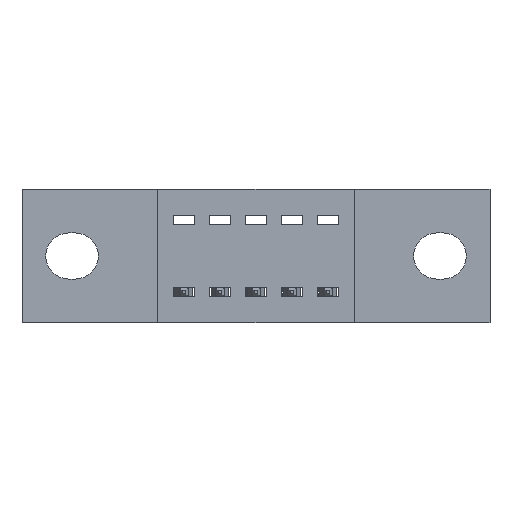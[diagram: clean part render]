
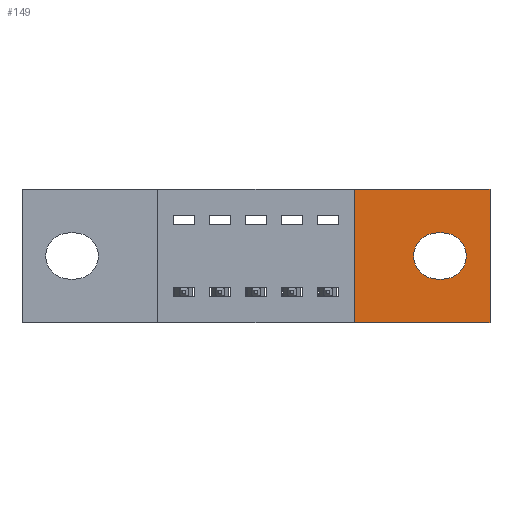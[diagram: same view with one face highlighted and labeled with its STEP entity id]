
A CAD part, front view. The second image highlights one B-rep face of the part: STEP entity #149.
In plain terms, the highlighted planar face has unit normal (0, -1, 0).
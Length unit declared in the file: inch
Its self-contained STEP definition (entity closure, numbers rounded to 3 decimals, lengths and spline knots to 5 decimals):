
#11 = DIRECTION ( 'NONE',  ( -1., 0., 0. ) ) ;
#149 = ADVANCED_FACE ( 'NONE', ( #6236, #7742 ), #6821, .T. ) ;
#252 = LINE ( 'NONE', #1247, #6644 ) ;
#316 = ORIENTED_EDGE ( 'NONE', *, *, #7622, .F. ) ;
#516 = CARTESIAN_POINT ( 'NONE',  ( 1.152, 0., -0.121 ) ) ;
#649 = AXIS2_PLACEMENT_3D ( 'NONE', #7775, #7868, #7463 ) ;
#774 = EDGE_CURVE ( 'NONE', #3691, #2990, #3386, .T. ) ;
#1015 = DIRECTION ( 'NONE',  ( 1., 0., 0. ) ) ;
#1027 = ORIENTED_EDGE ( 'NONE', *, *, #774, .T. ) ;
#1077 = EDGE_CURVE ( 'NONE', #6500, #5155, #3284, .T. ) ;
#1083 = VECTOR ( 'NONE', #11, 39.37008 ) ;
#1247 = CARTESIAN_POINT ( 'NONE',  ( 1.17, 0., -0.249 ) ) ;
#1268 = DIRECTION ( 'NONE',  ( -1., 0., 0. ) ) ;
#1325 = VECTOR ( 'NONE', #3061, 39.37008 ) ;
#1450 = CARTESIAN_POINT ( 'NONE',  ( 1.17, 0., -0.121 ) ) ;
#1493 = VECTOR ( 'NONE', #1015, 39.37008 ) ;
#1642 = CIRCLE ( 'NONE', #7330, 0.064 ) ;
#1705 = DIRECTION ( 'NONE',  ( 0., 0., 1. ) ) ;
#1780 = ORIENTED_EDGE ( 'NONE', *, *, #4935, .F. ) ;
#2041 = CARTESIAN_POINT ( 'NONE',  ( 0.923, 0., 0. ) ) ;
#2083 = VERTEX_POINT ( 'NONE', #2868 ) ;
#2131 = EDGE_CURVE ( 'NONE', #5155, #2083, #2318, .T. ) ;
#2318 = LINE ( 'NONE', #4399, #3565 ) ;
#2379 = CARTESIAN_POINT ( 'NONE',  ( 1.17, 0., -0.185 ) ) ;
#2868 = CARTESIAN_POINT ( 'NONE',  ( 1.3, 0., 0. ) ) ;
#2923 = EDGE_LOOP ( 'NONE', ( #1027, #7491, #4480, #3009 ) ) ;
#2990 = VERTEX_POINT ( 'NONE', #3347 ) ;
#3009 = ORIENTED_EDGE ( 'NONE', *, *, #3537, .T. ) ;
#3061 = DIRECTION ( 'NONE',  ( 0., 0., -1. ) ) ;
#3091 = CARTESIAN_POINT ( 'NONE',  ( 1.3, 0., 0. ) ) ;
#3123 = LINE ( 'NONE', #3091, #1325 ) ;
#3284 = LINE ( 'NONE', #5162, #6405 ) ;
#3317 = EDGE_LOOP ( 'NONE', ( #7819, #1780, #316, #3596 ) ) ;
#3347 = CARTESIAN_POINT ( 'NONE',  ( 1.17, 0., -0.249 ) ) ;
#3386 = CIRCLE ( 'NONE', #7445, 0.064 ) ;
#3406 = VERTEX_POINT ( 'NONE', #7368 ) ;
#3473 = VERTEX_POINT ( 'NONE', #516 ) ;
#3537 = EDGE_CURVE ( 'NONE', #3473, #3691, #7882, .T. ) ;
#3565 = VECTOR ( 'NONE', #6577, 39.37008 ) ;
#3577 = CARTESIAN_POINT ( 'NONE',  ( 0., 0., -0.37 ) ) ;
#3596 = ORIENTED_EDGE ( 'NONE', *, *, #2131, .F. ) ;
#3691 = VERTEX_POINT ( 'NONE', #6468 ) ;
#4213 = DIRECTION ( 'NONE',  ( 0., 1., 0. ) ) ;
#4399 = CARTESIAN_POINT ( 'NONE',  ( 0., 0., 0. ) ) ;
#4420 = CARTESIAN_POINT ( 'NONE',  ( 1.3, 0., -0.37 ) ) ;
#4480 = ORIENTED_EDGE ( 'NONE', *, *, #5614, .T. ) ;
#4597 = DIRECTION ( 'NONE',  ( 0., 0., -1. ) ) ;
#4606 = DIRECTION ( 'NONE',  ( 0., 1., 0. ) ) ;
#4608 = CARTESIAN_POINT ( 'NONE',  ( 1.152, 0., -0.185 ) ) ;
#4642 = CARTESIAN_POINT ( 'NONE',  ( 0.923, 0., -0.37 ) ) ;
#4935 = EDGE_CURVE ( 'NONE', #7365, #6500, #7540, .T. ) ;
#5155 = VERTEX_POINT ( 'NONE', #2041 ) ;
#5162 = CARTESIAN_POINT ( 'NONE',  ( 0.923, 0., -0.37 ) ) ;
#5573 = DIRECTION ( 'NONE',  ( 0., 0., -1. ) ) ;
#5614 = EDGE_CURVE ( 'NONE', #3406, #3473, #1642, .T. ) ;
#6236 = FACE_BOUND ( 'NONE', #2923, .T. ) ;
#6405 = VECTOR ( 'NONE', #1705, 39.37008 ) ;
#6468 = CARTESIAN_POINT ( 'NONE',  ( 1.17, 0., -0.121 ) ) ;
#6500 = VERTEX_POINT ( 'NONE', #4642 ) ;
#6577 = DIRECTION ( 'NONE',  ( 1., 0., 0. ) ) ;
#6644 = VECTOR ( 'NONE', #1268, 39.37008 ) ;
#6730 = EDGE_CURVE ( 'NONE', #2990, #3406, #252, .T. ) ;
#6821 = PLANE ( 'NONE',  #649 ) ;
#7330 = AXIS2_PLACEMENT_3D ( 'NONE', #4608, #4606, #4597 ) ;
#7365 = VERTEX_POINT ( 'NONE', #4420 ) ;
#7368 = CARTESIAN_POINT ( 'NONE',  ( 1.152, 0., -0.249 ) ) ;
#7445 = AXIS2_PLACEMENT_3D ( 'NONE', #2379, #4213, #5573 ) ;
#7463 = DIRECTION ( 'NONE',  ( 0., 0., -1. ) ) ;
#7491 = ORIENTED_EDGE ( 'NONE', *, *, #6730, .T. ) ;
#7540 = LINE ( 'NONE', #3577, #1083 ) ;
#7622 = EDGE_CURVE ( 'NONE', #2083, #7365, #3123, .T. ) ;
#7742 = FACE_OUTER_BOUND ( 'NONE', #3317, .T. ) ;
#7775 = CARTESIAN_POINT ( 'NONE',  ( 0., 0., -0.37 ) ) ;
#7819 = ORIENTED_EDGE ( 'NONE', *, *, #1077, .F. ) ;
#7868 = DIRECTION ( 'NONE',  ( 0., -1., 0. ) ) ;
#7882 = LINE ( 'NONE', #1450, #1493 ) ;
